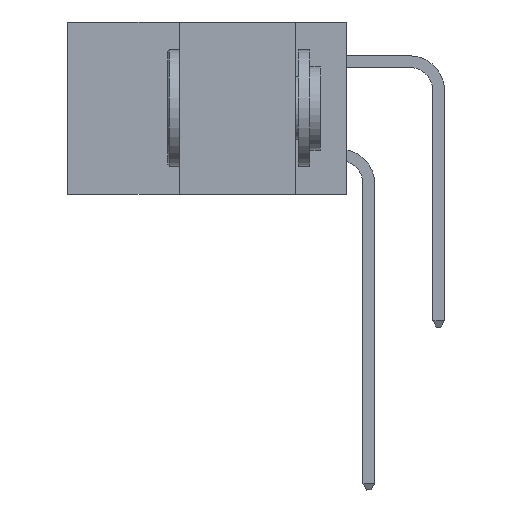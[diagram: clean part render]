
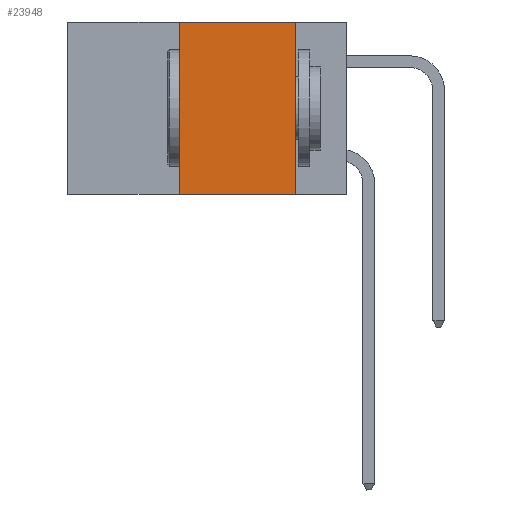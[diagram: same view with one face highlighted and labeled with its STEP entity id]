
A CAD part, left-side view. The second image highlights one B-rep face of the part: STEP entity #23948.
In plain terms, the highlighted planar face has unit normal (-1, 0, 0).
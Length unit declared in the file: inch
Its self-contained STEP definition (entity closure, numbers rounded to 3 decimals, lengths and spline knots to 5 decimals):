
#249 = CARTESIAN_POINT ( 'NONE',  ( 0., 0.6, 0. ) ) ;
#870 = LINE ( 'NONE', #8436, #17829 ) ;
#1945 = EDGE_CURVE ( 'NONE', #20848, #26369, #32275, .T. ) ;
#2366 = EDGE_CURVE ( 'NONE', #8185, #20848, #25964, .T. ) ;
#3555 = DIRECTION ( 'NONE',  ( 0., -1., 0. ) ) ;
#4732 = DIRECTION ( 'NONE',  ( 0., -1., 0. ) ) ;
#6035 = CARTESIAN_POINT ( 'NONE',  ( 0., 0.36, -0.37 ) ) ;
#7715 = ORIENTED_EDGE ( 'NONE', *, *, #17416, .T. ) ;
#8185 = VERTEX_POINT ( 'NONE', #27617 ) ;
#8436 = CARTESIAN_POINT ( 'NONE',  ( 0., 0.36, 0. ) ) ;
#11006 = CARTESIAN_POINT ( 'NONE',  ( 0., 0.11, 0. ) ) ;
#13466 = FACE_OUTER_BOUND ( 'NONE', #32531, .T. ) ;
#15613 = ORIENTED_EDGE ( 'NONE', *, *, #1945, .F. ) ;
#17355 = CARTESIAN_POINT ( 'NONE',  ( 0., 0.6, -0.37 ) ) ;
#17416 = EDGE_CURVE ( 'NONE', #21322, #26369, #38681, .T. ) ;
#17597 = ORIENTED_EDGE ( 'NONE', *, *, #2366, .F. ) ;
#17829 = VECTOR ( 'NONE', #33306, 39.37008 ) ;
#18200 = EDGE_CURVE ( 'NONE', #21322, #8185, #870, .T. ) ;
#18222 = DIRECTION ( 'NONE',  ( 1., 0., 0. ) ) ;
#20848 = VERTEX_POINT ( 'NONE', #35017 ) ;
#21322 = VERTEX_POINT ( 'NONE', #6035 ) ;
#21527 = ORIENTED_EDGE ( 'NONE', *, *, #18200, .F. ) ;
#23324 = CARTESIAN_POINT ( 'NONE',  ( 0., 0.11, -0.37 ) ) ;
#23948 = ADVANCED_FACE ( 'NONE', ( #13466 ), #36735, .F. ) ;
#24368 = CARTESIAN_POINT ( 'NONE',  ( 0., 0.6, 0. ) ) ;
#25964 = LINE ( 'NONE', #249, #26933 ) ;
#26369 = VERTEX_POINT ( 'NONE', #23324 ) ;
#26933 = VECTOR ( 'NONE', #3555, 39.37008 ) ;
#27617 = CARTESIAN_POINT ( 'NONE',  ( 0., 0.36, 0. ) ) ;
#29798 = DIRECTION ( 'NONE',  ( 0., 0., -1. ) ) ;
#31301 = VECTOR ( 'NONE', #29798, 39.37008 ) ;
#32275 = LINE ( 'NONE', #11006, #31301 ) ;
#32531 = EDGE_LOOP ( 'NONE', ( #15613, #17597, #21527, #7715 ) ) ;
#33306 = DIRECTION ( 'NONE',  ( 0., 0., 1. ) ) ;
#35017 = CARTESIAN_POINT ( 'NONE',  ( 0., 0.11, 0. ) ) ;
#35739 = AXIS2_PLACEMENT_3D ( 'NONE', #24368, #18222, #39844 ) ;
#36735 = PLANE ( 'NONE',  #35739 ) ;
#37714 = VECTOR ( 'NONE', #4732, 39.37008 ) ;
#38681 = LINE ( 'NONE', #17355, #37714 ) ;
#39844 = DIRECTION ( 'NONE',  ( 0., 0., -1. ) ) ;
